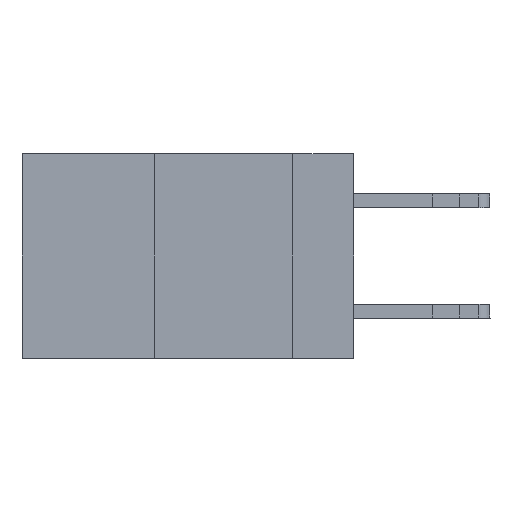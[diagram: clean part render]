
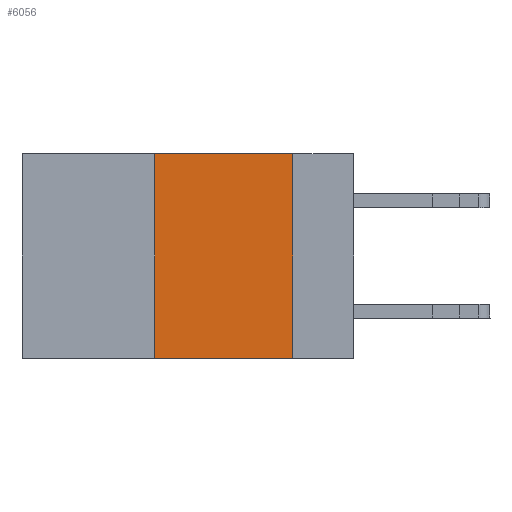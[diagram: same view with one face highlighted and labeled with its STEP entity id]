
A CAD part, left-side view. The second image highlights one B-rep face of the part: STEP entity #6056.
In plain terms, the highlighted planar face has unit normal (-1, 0, 0).
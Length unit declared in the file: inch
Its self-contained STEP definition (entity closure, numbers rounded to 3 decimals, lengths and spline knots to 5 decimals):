
#499 = CARTESIAN_POINT ( 'NONE',  ( 0., 0.11, 0. ) ) ;
#1568 = CARTESIAN_POINT ( 'NONE',  ( 0., 0.11, -0.37 ) ) ;
#3330 = FACE_OUTER_BOUND ( 'NONE', #22572, .T. ) ;
#3377 = VECTOR ( 'NONE', #21117, 39.37008 ) ;
#4108 = VERTEX_POINT ( 'NONE', #6558 ) ;
#4365 = EDGE_CURVE ( 'NONE', #24549, #13290, #27311, .T. ) ;
#4713 = ORIENTED_EDGE ( 'NONE', *, *, #25068, .F. ) ;
#4836 = PLANE ( 'NONE',  #7644 ) ;
#4856 = CARTESIAN_POINT ( 'NONE',  ( 0., 0.36, 0. ) ) ;
#5525 = EDGE_CURVE ( 'NONE', #4108, #15950, #9416, .T. ) ;
#6056 = ADVANCED_FACE ( 'NONE', ( #3330 ), #4836, .F. ) ;
#6558 = CARTESIAN_POINT ( 'NONE',  ( 0., 0.36, -0.37 ) ) ;
#7455 = VECTOR ( 'NONE', #11394, 39.37008 ) ;
#7644 = AXIS2_PLACEMENT_3D ( 'NONE', #15667, #9071, #19810 ) ;
#9071 = DIRECTION ( 'NONE',  ( 1., 0., 0. ) ) ;
#9081 = LINE ( 'NONE', #27328, #3377 ) ;
#9408 = ORIENTED_EDGE ( 'NONE', *, *, #19714, .F. ) ;
#9416 = LINE ( 'NONE', #9932, #20872 ) ;
#9932 = CARTESIAN_POINT ( 'NONE',  ( 0., 0.6, -0.37 ) ) ;
#11394 = DIRECTION ( 'NONE',  ( 0., 0., -1. ) ) ;
#11501 = DIRECTION ( 'NONE',  ( 0., -1., 0. ) ) ;
#11522 = ORIENTED_EDGE ( 'NONE', *, *, #5525, .T. ) ;
#13290 = VERTEX_POINT ( 'NONE', #18182 ) ;
#15561 = ORIENTED_EDGE ( 'NONE', *, *, #4365, .F. ) ;
#15667 = CARTESIAN_POINT ( 'NONE',  ( 0., 0.6, 0. ) ) ;
#15950 = VERTEX_POINT ( 'NONE', #1568 ) ;
#18182 = CARTESIAN_POINT ( 'NONE',  ( 0., 0.11, 0. ) ) ;
#19714 = EDGE_CURVE ( 'NONE', #4108, #24549, #9081, .T. ) ;
#19810 = DIRECTION ( 'NONE',  ( 0., 0., -1. ) ) ;
#19964 = CARTESIAN_POINT ( 'NONE',  ( 0., 0.6, 0. ) ) ;
#20872 = VECTOR ( 'NONE', #25170, 39.37008 ) ;
#21117 = DIRECTION ( 'NONE',  ( 0., 0., 1. ) ) ;
#22572 = EDGE_LOOP ( 'NONE', ( #4713, #15561, #9408, #11522 ) ) ;
#22598 = VECTOR ( 'NONE', #11501, 39.37008 ) ;
#24549 = VERTEX_POINT ( 'NONE', #4856 ) ;
#25068 = EDGE_CURVE ( 'NONE', #13290, #15950, #25272, .T. ) ;
#25170 = DIRECTION ( 'NONE',  ( 0., -1., 0. ) ) ;
#25272 = LINE ( 'NONE', #499, #7455 ) ;
#27311 = LINE ( 'NONE', #19964, #22598 ) ;
#27328 = CARTESIAN_POINT ( 'NONE',  ( 0., 0.36, 0. ) ) ;
